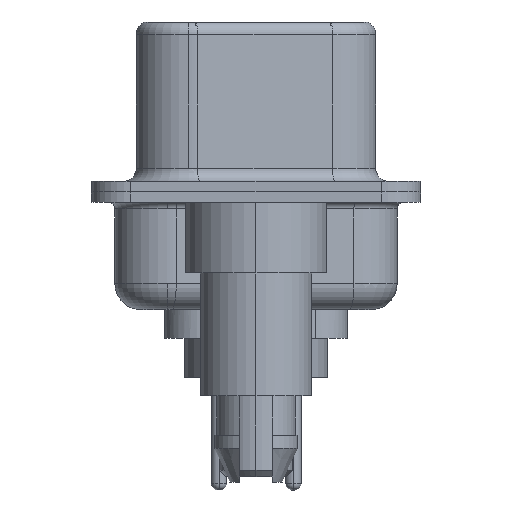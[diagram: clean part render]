
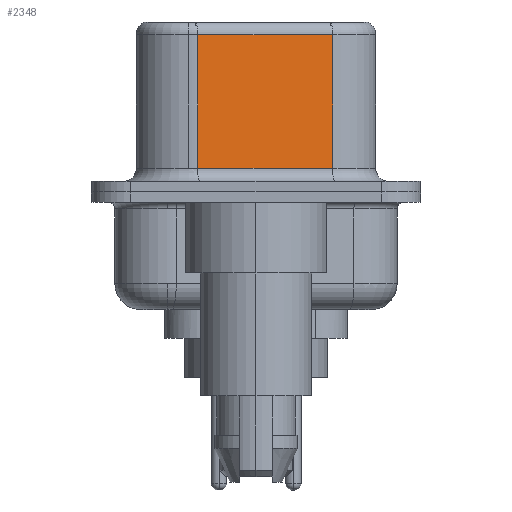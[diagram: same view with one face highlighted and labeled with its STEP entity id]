
A CAD part, left-side view. The second image highlights one B-rep face of the part: STEP entity #2348.
In plain terms, the highlighted planar face has unit normal (-0.985, -0.174, 0).
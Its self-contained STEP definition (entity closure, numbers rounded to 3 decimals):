
#16 = CARTESIAN_POINT ( 'NONE',  ( 4.58, -2.927, 6.52 ) ) ;
#743 = ORIENTED_EDGE ( 'NONE', *, *, #13345, .T. ) ;
#2348 = ADVANCED_FACE ( 'NONE', ( #12108 ), #11732, .F. ) ;
#3870 = VECTOR ( 'NONE', #15014, 1000. ) ;
#3934 = DIRECTION ( 'NONE',  ( 0., 0., -1. ) ) ;
#4137 = LINE ( 'NONE', #9866, #17447 ) ;
#4717 = LINE ( 'NONE', #18367, #23476 ) ;
#6092 = CARTESIAN_POINT ( 'NONE',  ( 4.58, -2.927, 0.9 ) ) ;
#7706 = VERTEX_POINT ( 'NONE', #11072 ) ;
#8797 = ORIENTED_EDGE ( 'NONE', *, *, #11427, .T. ) ;
#8825 = VERTEX_POINT ( 'NONE', #21371 ) ;
#9590 = DIRECTION ( 'NONE',  ( 0.985, 0.174, 0. ) ) ;
#9866 = CARTESIAN_POINT ( 'NONE',  ( 4.58, -2.927, 0.9 ) ) ;
#10943 = DIRECTION ( 'NONE',  ( 0., 0., -1. ) ) ;
#11072 = CARTESIAN_POINT ( 'NONE',  ( 3.67, 2.233, 0.9 ) ) ;
#11278 = VECTOR ( 'NONE', #10943, 1000. ) ;
#11417 = EDGE_LOOP ( 'NONE', ( #11840, #8797, #743, #15617 ) ) ;
#11427 = EDGE_CURVE ( 'NONE', #8825, #12820, #13517, .T. ) ;
#11732 = PLANE ( 'NONE',  #17848 ) ;
#11840 = ORIENTED_EDGE ( 'NONE', *, *, #13260, .F. ) ;
#12108 = FACE_OUTER_BOUND ( 'NONE', #11417, .T. ) ;
#12820 = VERTEX_POINT ( 'NONE', #16947 ) ;
#12821 = VERTEX_POINT ( 'NONE', #6092 ) ;
#13260 = EDGE_CURVE ( 'NONE', #8825, #12821, #20899, .T. ) ;
#13345 = EDGE_CURVE ( 'NONE', #12820, #7706, #4717, .T. ) ;
#13517 = LINE ( 'NONE', #16841, #3870 ) ;
#14000 = EDGE_CURVE ( 'NONE', #7706, #12821, #4137, .T. ) ;
#15014 = DIRECTION ( 'NONE',  ( -0.174, 0.985, 0. ) ) ;
#15617 = ORIENTED_EDGE ( 'NONE', *, *, #14000, .T. ) ;
#15669 = CARTESIAN_POINT ( 'NONE',  ( 4.58, -2.927, 6.52 ) ) ;
#16841 = CARTESIAN_POINT ( 'NONE',  ( 4.58, -2.927, 6.02 ) ) ;
#16947 = CARTESIAN_POINT ( 'NONE',  ( 3.67, 2.233, 6.02 ) ) ;
#17447 = VECTOR ( 'NONE', #22534, 1000. ) ;
#17848 = AXIS2_PLACEMENT_3D ( 'NONE', #15669, #9590, #20503 ) ;
#18367 = CARTESIAN_POINT ( 'NONE',  ( 3.67, 2.233, 6.52 ) ) ;
#20503 = DIRECTION ( 'NONE',  ( -0.174, 0.985, 0. ) ) ;
#20899 = LINE ( 'NONE', #16, #11278 ) ;
#21371 = CARTESIAN_POINT ( 'NONE',  ( 4.58, -2.927, 6.02 ) ) ;
#22534 = DIRECTION ( 'NONE',  ( 0.174, -0.985, 0. ) ) ;
#23476 = VECTOR ( 'NONE', #3934, 1000. ) ;
